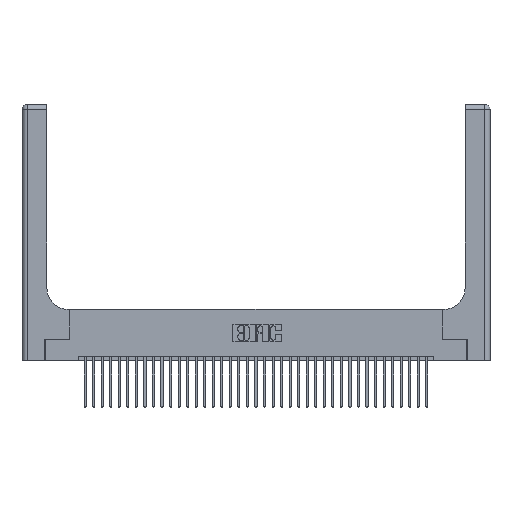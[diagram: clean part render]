
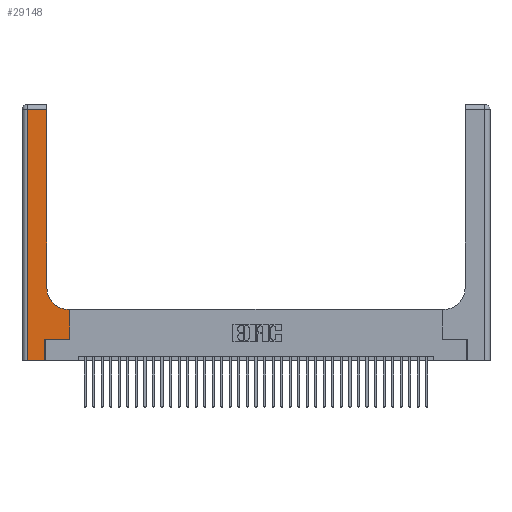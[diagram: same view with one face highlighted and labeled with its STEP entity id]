
A CAD part, top view. The second image highlights one B-rep face of the part: STEP entity #29148.
In plain terms, the highlighted planar face has unit normal (0, 0, 1).
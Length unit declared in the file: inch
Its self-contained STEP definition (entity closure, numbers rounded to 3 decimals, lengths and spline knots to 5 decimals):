
#576 = CARTESIAN_POINT ( 'NONE',  ( 0.5585, 0.25, 0.37 ) ) ;
#1338 = VECTOR ( 'NONE', #23330, 39.37008 ) ;
#2003 = VERTEX_POINT ( 'NONE', #32138 ) ;
#2192 = DIRECTION ( 'NONE',  ( 0., -1., 0. ) ) ;
#2210 = CIRCLE ( 'NONE', #3978, 0.25 ) ;
#2387 = CARTESIAN_POINT ( 'NONE',  ( 0.2915, 3., 0.37 ) ) ;
#2907 = VECTOR ( 'NONE', #2192, 39.37008 ) ;
#3062 = VECTOR ( 'NONE', #12517, 39.37008 ) ;
#3469 = VECTOR ( 'NONE', #28967, 39.37008 ) ;
#3978 = AXIS2_PLACEMENT_3D ( 'NONE', #4945, #5201, #36833 ) ;
#4002 = LINE ( 'NONE', #22930, #3062 ) ;
#4425 = DIRECTION ( 'NONE',  ( 1., 0., 0. ) ) ;
#4945 = CARTESIAN_POINT ( 'NONE',  ( 0.5415, 0.85, 0.37 ) ) ;
#5045 = LINE ( 'NONE', #24558, #28138 ) ;
#5201 = DIRECTION ( 'NONE',  ( 0., 0., -1. ) ) ;
#5715 = EDGE_CURVE ( 'NONE', #22025, #13233, #19277, .T. ) ;
#5879 = ORIENTED_EDGE ( 'NONE', *, *, #35896, .T. ) ;
#5932 = VERTEX_POINT ( 'NONE', #6399 ) ;
#6399 = CARTESIAN_POINT ( 'NONE',  ( 0.2915, 0.85, 0.37 ) ) ;
#6724 = VECTOR ( 'NONE', #29680, 39.37008 ) ;
#9119 = LINE ( 'NONE', #26192, #12699 ) ;
#9320 = CARTESIAN_POINT ( 'NONE',  ( 0.5585, 0.6, 0.37 ) ) ;
#9964 = LINE ( 'NONE', #11928, #1338 ) ;
#10382 = AXIS2_PLACEMENT_3D ( 'NONE', #27059, #12603, #15261 ) ;
#10385 = EDGE_CURVE ( 'NONE', #10851, #2003, #9964, .T. ) ;
#10613 = ORIENTED_EDGE ( 'NONE', *, *, #20315, .T. ) ;
#10851 = VERTEX_POINT ( 'NONE', #37409 ) ;
#11427 = ORIENTED_EDGE ( 'NONE', *, *, #10385, .T. ) ;
#11928 = CARTESIAN_POINT ( 'NONE',  ( 0., 0., 0.37 ) ) ;
#12217 = EDGE_LOOP ( 'NONE', ( #5879, #33852, #18886, #11427, #18768, #22184, #25142, #10613, #20477 ) ) ;
#12517 = DIRECTION ( 'NONE',  ( -1., 0., 0. ) ) ;
#12603 = DIRECTION ( 'NONE',  ( 0., 0., -1. ) ) ;
#12699 = VECTOR ( 'NONE', #23545, 39.37008 ) ;
#13233 = VERTEX_POINT ( 'NONE', #27244 ) ;
#14350 = LINE ( 'NONE', #20699, #6724 ) ;
#14747 = CARTESIAN_POINT ( 'NONE',  ( 0.5415, 0.6, 0.37 ) ) ;
#14957 = EDGE_CURVE ( 'NONE', #30764, #29712, #5045, .T. ) ;
#15261 = DIRECTION ( 'NONE',  ( -1., 0., 0. ) ) ;
#17585 = LINE ( 'NONE', #2387, #23502 ) ;
#18768 = ORIENTED_EDGE ( 'NONE', *, *, #30905, .T. ) ;
#18886 = ORIENTED_EDGE ( 'NONE', *, *, #32549, .T. ) ;
#19277 = LINE ( 'NONE', #23155, #3469 ) ;
#20315 = EDGE_CURVE ( 'NONE', #32736, #32175, #4002, .T. ) ;
#20477 = ORIENTED_EDGE ( 'NONE', *, *, #35813, .T. ) ;
#20699 = CARTESIAN_POINT ( 'NONE',  ( 0.269, 0., 0.37 ) ) ;
#20740 = PLANE ( 'NONE',  #10382 ) ;
#22025 = VERTEX_POINT ( 'NONE', #24424 ) ;
#22184 = ORIENTED_EDGE ( 'NONE', *, *, #14957, .T. ) ;
#22930 = CARTESIAN_POINT ( 'NONE',  ( 0.2915, 0.6, 0.37 ) ) ;
#23155 = CARTESIAN_POINT ( 'NONE',  ( 0., 2.94, 0.37 ) ) ;
#23330 = DIRECTION ( 'NONE',  ( 1., 0., 0. ) ) ;
#23502 = VECTOR ( 'NONE', #31250, 39.37008 ) ;
#23545 = DIRECTION ( 'NONE',  ( 0., 1., 0. ) ) ;
#23725 = EDGE_CURVE ( 'NONE', #29712, #32736, #9119, .T. ) ;
#24424 = CARTESIAN_POINT ( 'NONE',  ( 0.2915, 2.94, 0.37 ) ) ;
#24558 = CARTESIAN_POINT ( 'NONE',  ( 0.269, 0.25, 0.37 ) ) ;
#25142 = ORIENTED_EDGE ( 'NONE', *, *, #23725, .T. ) ;
#26143 = CARTESIAN_POINT ( 'NONE',  ( 0.269, 0.25, 0.37 ) ) ;
#26192 = CARTESIAN_POINT ( 'NONE',  ( 0.5585, 0.25, 0.37 ) ) ;
#27059 = CARTESIAN_POINT ( 'NONE',  ( 0., 3., 0.37 ) ) ;
#27244 = CARTESIAN_POINT ( 'NONE',  ( 0.06, 2.94, 0.37 ) ) ;
#27808 = LINE ( 'NONE', #31174, #2907 ) ;
#28138 = VECTOR ( 'NONE', #4425, 39.37008 ) ;
#28967 = DIRECTION ( 'NONE',  ( -1., 0., 0. ) ) ;
#29148 = ADVANCED_FACE ( 'NONE', ( #35000 ), #20740, .F. ) ;
#29680 = DIRECTION ( 'NONE',  ( 0., 1., 0. ) ) ;
#29712 = VERTEX_POINT ( 'NONE', #576 ) ;
#30764 = VERTEX_POINT ( 'NONE', #26143 ) ;
#30905 = EDGE_CURVE ( 'NONE', #2003, #30764, #14350, .T. ) ;
#31174 = CARTESIAN_POINT ( 'NONE',  ( 0.06, 3., 0.37 ) ) ;
#31250 = DIRECTION ( 'NONE',  ( 0., 1., 0. ) ) ;
#32138 = CARTESIAN_POINT ( 'NONE',  ( 0.269, 0., 0.37 ) ) ;
#32175 = VERTEX_POINT ( 'NONE', #14747 ) ;
#32549 = EDGE_CURVE ( 'NONE', #13233, #10851, #27808, .T. ) ;
#32736 = VERTEX_POINT ( 'NONE', #9320 ) ;
#33852 = ORIENTED_EDGE ( 'NONE', *, *, #5715, .T. ) ;
#35000 = FACE_OUTER_BOUND ( 'NONE', #12217, .T. ) ;
#35813 = EDGE_CURVE ( 'NONE', #32175, #5932, #2210, .T. ) ;
#35896 = EDGE_CURVE ( 'NONE', #5932, #22025, #17585, .T. ) ;
#36833 = DIRECTION ( 'NONE',  ( 1., 0., 0. ) ) ;
#37409 = CARTESIAN_POINT ( 'NONE',  ( 0.06, 0., 0.37 ) ) ;
